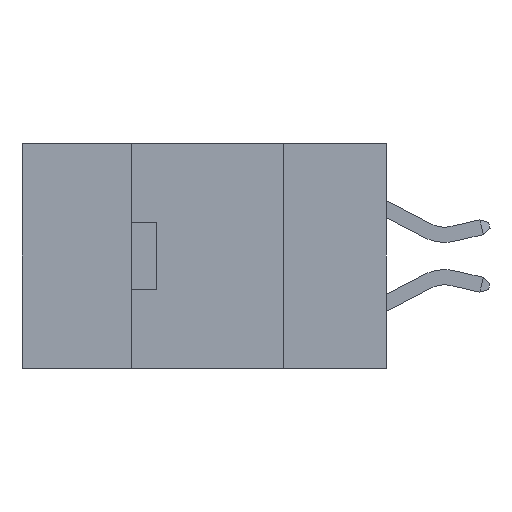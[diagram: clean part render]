
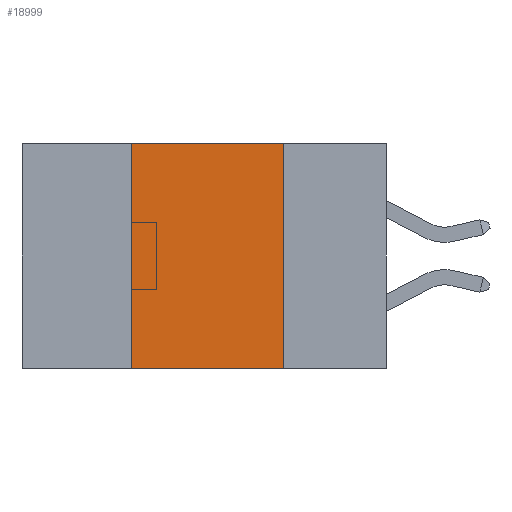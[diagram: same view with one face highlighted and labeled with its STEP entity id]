
A CAD part, left-side view. The second image highlights one B-rep face of the part: STEP entity #18999.
In plain terms, the highlighted planar face has unit normal (-1, 0, 0).
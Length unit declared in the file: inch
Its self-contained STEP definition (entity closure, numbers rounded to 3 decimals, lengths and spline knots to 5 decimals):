
#267 = DIRECTION ( 'NONE',  ( 0., 0., -1. ) ) ;
#1094 = VERTEX_POINT ( 'NONE', #3712 ) ;
#1311 = DIRECTION ( 'NONE',  ( 0., -1., 0. ) ) ;
#1460 = DIRECTION ( 'NONE',  ( 0., 0., 1. ) ) ;
#1516 = CARTESIAN_POINT ( 'NONE',  ( 0., 0.17, 0. ) ) ;
#1810 = AXIS2_PLACEMENT_3D ( 'NONE', #10643, #26019, #12860 ) ;
#3554 = LINE ( 'NONE', #7919, #9476 ) ;
#3712 = CARTESIAN_POINT ( 'NONE',  ( 0., 0.42, -0.37 ) ) ;
#4572 = FACE_OUTER_BOUND ( 'NONE', #8916, .T. ) ;
#4821 = ORIENTED_EDGE ( 'NONE', *, *, #19582, .F. ) ;
#5498 = CARTESIAN_POINT ( 'NONE',  ( 0., 0.6, 0. ) ) ;
#6159 = PLANE ( 'NONE',  #1810 ) ;
#6521 = CARTESIAN_POINT ( 'NONE',  ( 0., 0.17, -0.37 ) ) ;
#7919 = CARTESIAN_POINT ( 'NONE',  ( 0., 0.6, -0.37 ) ) ;
#8062 = VECTOR ( 'NONE', #16607, 39.37008 ) ;
#8916 = EDGE_LOOP ( 'NONE', ( #26231, #21834, #4821, #10774 ) ) ;
#9476 = VECTOR ( 'NONE', #1311, 39.37008 ) ;
#10505 = VERTEX_POINT ( 'NONE', #16557 ) ;
#10643 = CARTESIAN_POINT ( 'NONE',  ( 0., 0.6, 0. ) ) ;
#10774 = ORIENTED_EDGE ( 'NONE', *, *, #18093, .T. ) ;
#10828 = LINE ( 'NONE', #12544, #28329 ) ;
#11441 = VERTEX_POINT ( 'NONE', #1516 ) ;
#12286 = VERTEX_POINT ( 'NONE', #6521 ) ;
#12544 = CARTESIAN_POINT ( 'NONE',  ( 0., 0.42, -0.37 ) ) ;
#12860 = DIRECTION ( 'NONE',  ( 0., 0., -1. ) ) ;
#15391 = LINE ( 'NONE', #5498, #8062 ) ;
#15638 = LINE ( 'NONE', #15857, #22164 ) ;
#15857 = CARTESIAN_POINT ( 'NONE',  ( 0., 0.17, -0.37 ) ) ;
#16557 = CARTESIAN_POINT ( 'NONE',  ( 0., 0.42, 0. ) ) ;
#16607 = DIRECTION ( 'NONE',  ( 0., -1., 0. ) ) ;
#18093 = EDGE_CURVE ( 'NONE', #1094, #12286, #3554, .T. ) ;
#18999 = ADVANCED_FACE ( 'NONE', ( #4572 ), #6159, .F. ) ;
#19582 = EDGE_CURVE ( 'NONE', #1094, #10505, #10828, .T. ) ;
#21834 = ORIENTED_EDGE ( 'NONE', *, *, #23945, .F. ) ;
#22164 = VECTOR ( 'NONE', #267, 39.37008 ) ;
#23945 = EDGE_CURVE ( 'NONE', #10505, #11441, #15391, .T. ) ;
#25385 = EDGE_CURVE ( 'NONE', #11441, #12286, #15638, .T. ) ;
#26019 = DIRECTION ( 'NONE',  ( 1., 0., 0. ) ) ;
#26231 = ORIENTED_EDGE ( 'NONE', *, *, #25385, .F. ) ;
#28329 = VECTOR ( 'NONE', #1460, 39.37008 ) ;
